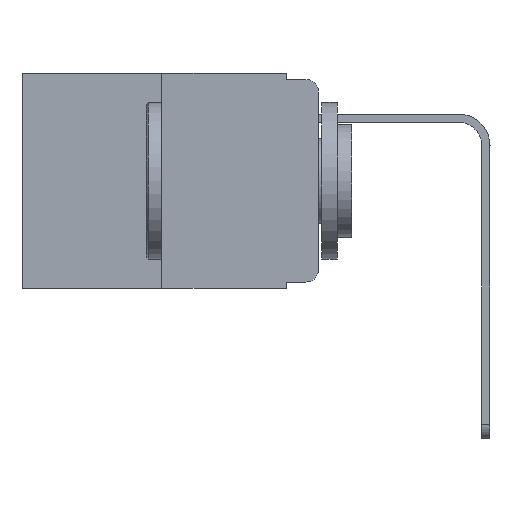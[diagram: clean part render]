
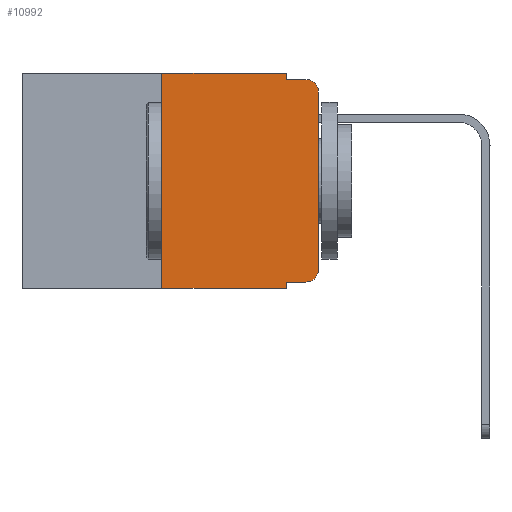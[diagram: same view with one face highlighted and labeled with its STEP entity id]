
A CAD part, left-side view. The second image highlights one B-rep face of the part: STEP entity #10992.
In plain terms, the highlighted planar face has unit normal (-1, 0, 0).
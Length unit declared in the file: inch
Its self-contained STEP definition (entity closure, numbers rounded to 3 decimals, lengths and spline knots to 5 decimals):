
#7 = AXIS2_PLACEMENT_3D ( 'NONE', #1903, #10529, #12965 ) ;
#231 = CARTESIAN_POINT ( 'NONE',  ( 0., 0.051, -0.343 ) ) ;
#248 = ORIENTED_EDGE ( 'NONE', *, *, #12405, .F. ) ;
#380 = CARTESIAN_POINT ( 'NONE',  ( 0., 0.02, -0.333 ) ) ;
#659 = ORIENTED_EDGE ( 'NONE', *, *, #1649, .T. ) ;
#661 = VERTEX_POINT ( 'NONE', #13603 ) ;
#1202 = VECTOR ( 'NONE', #6221, 39.37008 ) ;
#1217 = PLANE ( 'NONE',  #5351 ) ;
#1354 = DIRECTION ( 'NONE',  ( -1., 0., 0. ) ) ;
#1649 = EDGE_CURVE ( 'NONE', #8660, #2239, #11963, .T. ) ;
#1833 = LINE ( 'NONE', #10513, #4166 ) ;
#1854 = VERTEX_POINT ( 'NONE', #231 ) ;
#1899 = DIRECTION ( 'NONE',  ( 0., -1., 0. ) ) ;
#1903 = CARTESIAN_POINT ( 'NONE',  ( 0., 0.02, -0.313 ) ) ;
#2005 = ORIENTED_EDGE ( 'NONE', *, *, #13446, .T. ) ;
#2147 = CIRCLE ( 'NONE', #7, 0.02 ) ;
#2239 = VERTEX_POINT ( 'NONE', #6050 ) ;
#2290 = LINE ( 'NONE', #14992, #9052 ) ;
#2440 = ORIENTED_EDGE ( 'NONE', *, *, #12115, .T. ) ;
#2499 = DIRECTION ( 'NONE',  ( 1., 0., 0. ) ) ;
#2589 = VERTEX_POINT ( 'NONE', #7631 ) ;
#2725 = EDGE_CURVE ( 'NONE', #12401, #2239, #1833, .T. ) ;
#3756 = CARTESIAN_POINT ( 'NONE',  ( 0., 0.051, -0.333 ) ) ;
#3928 = LINE ( 'NONE', #15812, #8939 ) ;
#4166 = VECTOR ( 'NONE', #15371, 39.37008 ) ;
#4277 = EDGE_CURVE ( 'NONE', #14365, #661, #2147, .T. ) ;
#4523 = DIRECTION ( 'NONE',  ( 0., -1., 0. ) ) ;
#4662 = LINE ( 'NONE', #15551, #7904 ) ;
#5351 = AXIS2_PLACEMENT_3D ( 'NONE', #11124, #2499, #9829 ) ;
#5515 = LINE ( 'NONE', #14183, #10882 ) ;
#5550 = VERTEX_POINT ( 'NONE', #6714 ) ;
#5661 = CARTESIAN_POINT ( 'NONE',  ( 0., 0.473, -0.343 ) ) ;
#5860 = LINE ( 'NONE', #3756, #1202 ) ;
#5883 = ORIENTED_EDGE ( 'NONE', *, *, #7796, .T. ) ;
#6050 = CARTESIAN_POINT ( 'NONE',  ( 0., 0.02, -0.01 ) ) ;
#6221 = DIRECTION ( 'NONE',  ( 0., -1., 0. ) ) ;
#6628 = LINE ( 'NONE', #5661, #12759 ) ;
#6636 = CARTESIAN_POINT ( 'NONE',  ( 0., 0.051, 0. ) ) ;
#6714 = CARTESIAN_POINT ( 'NONE',  ( 0., 0.051, 0. ) ) ;
#6816 = DIRECTION ( 'NONE',  ( 0., 0., 1. ) ) ;
#6925 = EDGE_CURVE ( 'NONE', #10380, #5550, #5515, .T. ) ;
#7231 = VECTOR ( 'NONE', #10240, 39.37008 ) ;
#7373 = CARTESIAN_POINT ( 'NONE',  ( 0., 0.25, 0. ) ) ;
#7466 = VERTEX_POINT ( 'NONE', #8218 ) ;
#7631 = CARTESIAN_POINT ( 'NONE',  ( 0., 0.051, -0.333 ) ) ;
#7667 = EDGE_CURVE ( 'NONE', #7466, #10380, #3928, .T. ) ;
#7796 = EDGE_CURVE ( 'NONE', #2589, #14365, #5860, .T. ) ;
#7904 = VECTOR ( 'NONE', #6816, 39.37008 ) ;
#7990 = ORIENTED_EDGE ( 'NONE', *, *, #11356, .F. ) ;
#8135 = ORIENTED_EDGE ( 'NONE', *, *, #2725, .F. ) ;
#8218 = CARTESIAN_POINT ( 'NONE',  ( 0., 0.25, -0.343 ) ) ;
#8660 = VERTEX_POINT ( 'NONE', #9668 ) ;
#8670 = ORIENTED_EDGE ( 'NONE', *, *, #7667, .F. ) ;
#8761 = EDGE_LOOP ( 'NONE', ( #2005, #659, #8135, #248, #9869, #8670, #2440, #7990, #5883, #14835 ) ) ;
#8939 = VECTOR ( 'NONE', #13409, 39.37008 ) ;
#9032 = CARTESIAN_POINT ( 'NONE',  ( 0., 0.051, -0.01 ) ) ;
#9052 = VECTOR ( 'NONE', #13934, 39.37008 ) ;
#9570 = FACE_OUTER_BOUND ( 'NONE', #8761, .T. ) ;
#9668 = CARTESIAN_POINT ( 'NONE',  ( 0., 0., -0.03 ) ) ;
#9829 = DIRECTION ( 'NONE',  ( 0., 0., -1. ) ) ;
#9869 = ORIENTED_EDGE ( 'NONE', *, *, #6925, .F. ) ;
#10117 = LINE ( 'NONE', #6636, #7231 ) ;
#10240 = DIRECTION ( 'NONE',  ( 0., 0., -1. ) ) ;
#10380 = VERTEX_POINT ( 'NONE', #7373 ) ;
#10513 = CARTESIAN_POINT ( 'NONE',  ( 0., 0.051, -0.01 ) ) ;
#10529 = DIRECTION ( 'NONE',  ( -1., 0., 0. ) ) ;
#10882 = VECTOR ( 'NONE', #1899, 39.37008 ) ;
#10992 = ADVANCED_FACE ( 'NONE', ( #9570 ), #1217, .F. ) ;
#11124 = CARTESIAN_POINT ( 'NONE',  ( 0., 0.473, 0. ) ) ;
#11356 = EDGE_CURVE ( 'NONE', #2589, #1854, #10117, .T. ) ;
#11963 = CIRCLE ( 'NONE', #15188, 0.02 ) ;
#12115 = EDGE_CURVE ( 'NONE', #7466, #1854, #6628, .T. ) ;
#12216 = DIRECTION ( 'NONE',  ( 0., 0., -1. ) ) ;
#12401 = VERTEX_POINT ( 'NONE', #9032 ) ;
#12405 = EDGE_CURVE ( 'NONE', #5550, #12401, #2290, .T. ) ;
#12759 = VECTOR ( 'NONE', #4523, 39.37008 ) ;
#12965 = DIRECTION ( 'NONE',  ( 0., 0., -1. ) ) ;
#13409 = DIRECTION ( 'NONE',  ( 0., 0., 1. ) ) ;
#13446 = EDGE_CURVE ( 'NONE', #661, #8660, #4662, .T. ) ;
#13554 = CARTESIAN_POINT ( 'NONE',  ( 0., 0.02, -0.03 ) ) ;
#13603 = CARTESIAN_POINT ( 'NONE',  ( 0., 0., -0.313 ) ) ;
#13934 = DIRECTION ( 'NONE',  ( 0., 0., -1. ) ) ;
#14183 = CARTESIAN_POINT ( 'NONE',  ( 0., 0.473, 0. ) ) ;
#14365 = VERTEX_POINT ( 'NONE', #380 ) ;
#14835 = ORIENTED_EDGE ( 'NONE', *, *, #4277, .T. ) ;
#14992 = CARTESIAN_POINT ( 'NONE',  ( 0., 0.051, 0. ) ) ;
#15188 = AXIS2_PLACEMENT_3D ( 'NONE', #13554, #1354, #12216 ) ;
#15371 = DIRECTION ( 'NONE',  ( 0., -1., 0. ) ) ;
#15551 = CARTESIAN_POINT ( 'NONE',  ( 0., 0., 0. ) ) ;
#15812 = CARTESIAN_POINT ( 'NONE',  ( 0., 0.25, 0. ) ) ;
